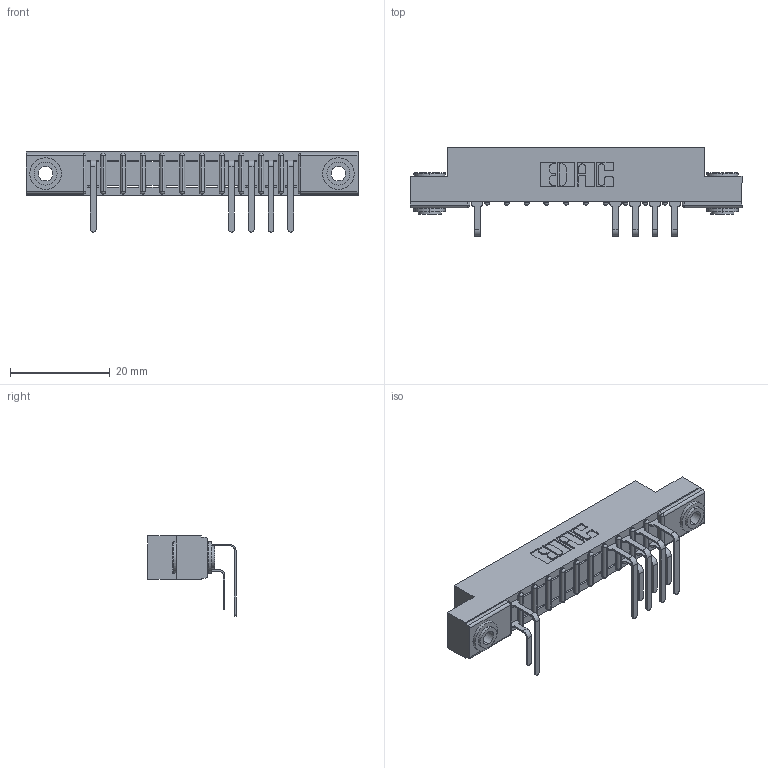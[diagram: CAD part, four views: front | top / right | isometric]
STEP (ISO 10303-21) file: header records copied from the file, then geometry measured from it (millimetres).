
FILE_DESCRIPTION (( 'STEP AP203' ), '1' );
FILE_NAME ('307-022-559-203.STEP', '2018-08-04T04:35:08', ( '' ), ( '' ), 'SwSTEP 2.0', 'SolidWorks 2016', '' );
FILE_SCHEMA (( 'CONFIG_CONTROL_DESIGN' ));
Length unit declared in the file: inch
Products named in the file (5): 307 Part_.156 Dia Mounting Holes; 307-290-001_558 559 - 1 (Single); 307-290-001_559 - 2 (Single); 345-250-002_345-250-002-102; 307-022-559-203
Assembly tree (12 placements, depth 2):
  307-022-559-203
    307 Part_.156 Dia Mounting Holes
    307-290-001_558 559 - 1 (Single)  x4
    307-290-001_559 - 2 (Single)  x5
    345-250-002_345-250-002-102  x2
Bounding box: 66.6 x 17.69 x 16.08 mm (x, y, z)
Volume: 4232 mm3; surface area: 6389.1 mm2
Topology: 12 solids, 12 shells, 762 faces, 2129 edges, 1370 vertices
Faces by surface type: plane 469, cylinder 261, sphere 24, cone 8
Entity records: 15700 total; most frequent: CARTESIAN_POINT 2617, ORIENTED_EDGE 2594, DIRECTION 2577, EDGE_CURVE 1297, LINE 973, VECTOR 973, VERTEX_POINT 842, AXIS2_PLACEMENT_3D 802
